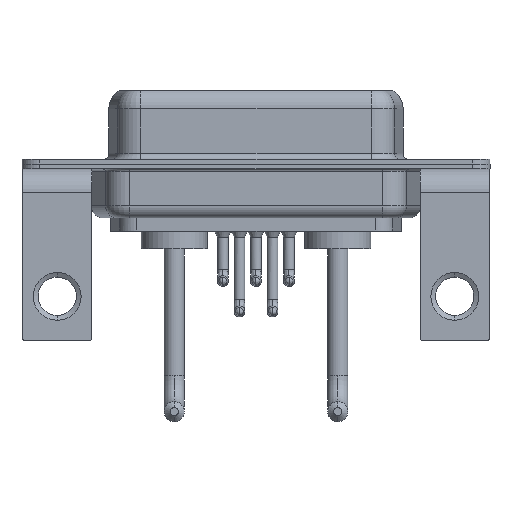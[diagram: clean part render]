
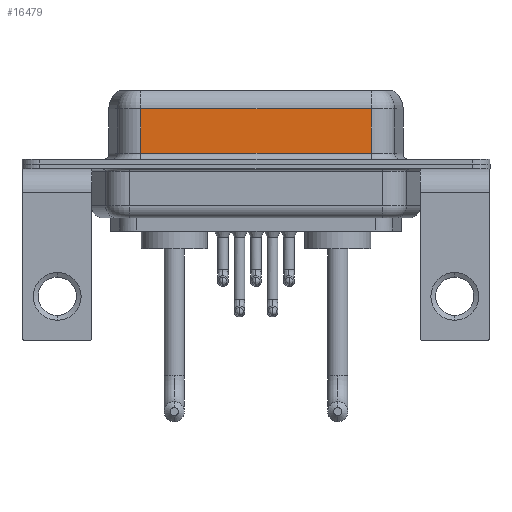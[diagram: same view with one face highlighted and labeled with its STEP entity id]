
A CAD part, front view. The second image highlights one B-rep face of the part: STEP entity #16479.
In plain terms, the highlighted planar face has unit normal (0, -1, 0).
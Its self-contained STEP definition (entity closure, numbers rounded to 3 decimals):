
#381 = CARTESIAN_POINT ( 'NONE',  ( 7.013, -3.95, 0.9 ) ) ;
#407 = ORIENTED_EDGE ( 'NONE', *, *, #3478, .F. ) ;
#617 = DIRECTION ( 'NONE',  ( -1., 0., 0. ) ) ;
#740 = ORIENTED_EDGE ( 'NONE', *, *, #13919, .T. ) ;
#1380 = VERTEX_POINT ( 'NONE', #8115 ) ;
#1603 = DIRECTION ( 'NONE',  ( 1., 0., 0. ) ) ;
#2015 = VERTEX_POINT ( 'NONE', #381 ) ;
#2347 = LINE ( 'NONE', #16195, #17136 ) ;
#3084 = CARTESIAN_POINT ( 'NONE',  ( 7.013, -3.95, 6.4 ) ) ;
#3478 = EDGE_CURVE ( 'NONE', #1380, #16800, #2347, .T. ) ;
#4555 = LINE ( 'NONE', #9039, #14654 ) ;
#5640 = EDGE_CURVE ( 'NONE', #1380, #8263, #4555, .T. ) ;
#5807 = CARTESIAN_POINT ( 'NONE',  ( 7.013, -3.95, 4.65 ) ) ;
#6924 = DIRECTION ( 'NONE',  ( 0., 0., -1. ) ) ;
#7596 = AXIS2_PLACEMENT_3D ( 'NONE', #16286, #13706, #9617 ) ;
#8115 = CARTESIAN_POINT ( 'NONE',  ( 26.287, -3.95, 4.65 ) ) ;
#8263 = VERTEX_POINT ( 'NONE', #5807 ) ;
#8497 = LINE ( 'NONE', #11187, #10529 ) ;
#9039 = CARTESIAN_POINT ( 'NONE',  ( 26.287, -3.95, 4.65 ) ) ;
#9067 = CARTESIAN_POINT ( 'NONE',  ( 26.287, -3.95, 0.9 ) ) ;
#9245 = DIRECTION ( 'NONE',  ( 0., 0., -1. ) ) ;
#9617 = DIRECTION ( 'NONE',  ( 0., 0., 1. ) ) ;
#9798 = LINE ( 'NONE', #3084, #14083 ) ;
#10326 = EDGE_CURVE ( 'NONE', #2015, #16800, #8497, .T. ) ;
#10529 = VECTOR ( 'NONE', #1603, 1000. ) ;
#10834 = ORIENTED_EDGE ( 'NONE', *, *, #5640, .T. ) ;
#11187 = CARTESIAN_POINT ( 'NONE',  ( 26.287, -3.95, 0.9 ) ) ;
#13286 = EDGE_LOOP ( 'NONE', ( #407, #10834, #740, #16581 ) ) ;
#13706 = DIRECTION ( 'NONE',  ( 0., 1., 0. ) ) ;
#13887 = FACE_OUTER_BOUND ( 'NONE', #13286, .T. ) ;
#13919 = EDGE_CURVE ( 'NONE', #8263, #2015, #9798, .T. ) ;
#14083 = VECTOR ( 'NONE', #6924, 1000. ) ;
#14654 = VECTOR ( 'NONE', #617, 1000. ) ;
#16195 = CARTESIAN_POINT ( 'NONE',  ( 26.287, -3.95, 6.4 ) ) ;
#16286 = CARTESIAN_POINT ( 'NONE',  ( 26.287, -3.95, 6.4 ) ) ;
#16479 = ADVANCED_FACE ( 'NONE', ( #13887 ), #17616, .F. ) ;
#16581 = ORIENTED_EDGE ( 'NONE', *, *, #10326, .T. ) ;
#16800 = VERTEX_POINT ( 'NONE', #9067 ) ;
#17136 = VECTOR ( 'NONE', #9245, 1000. ) ;
#17616 = PLANE ( 'NONE',  #7596 ) ;
